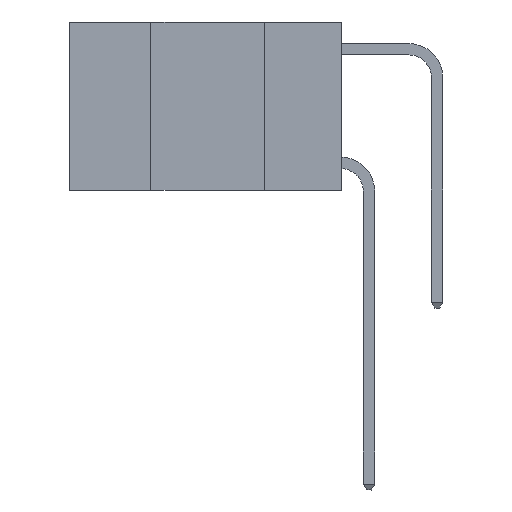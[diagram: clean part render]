
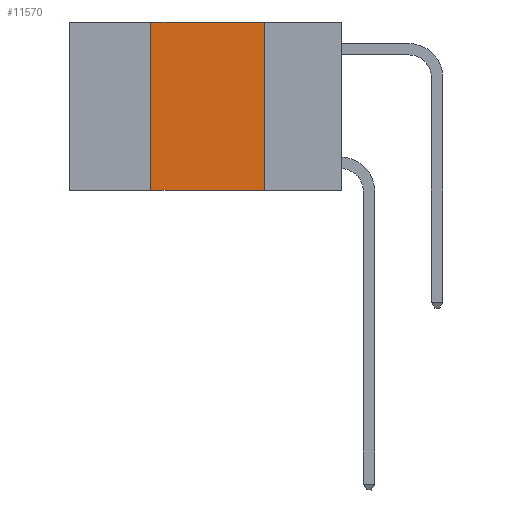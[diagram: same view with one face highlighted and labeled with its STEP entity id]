
A CAD part, left-side view. The second image highlights one B-rep face of the part: STEP entity #11570.
In plain terms, the highlighted planar face has unit normal (-1, 0, 0).
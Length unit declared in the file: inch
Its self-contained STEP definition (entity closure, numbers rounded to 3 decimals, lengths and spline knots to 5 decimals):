
#505 = VERTEX_POINT ( 'NONE', #12590 ) ;
#837 = VERTEX_POINT ( 'NONE', #8131 ) ;
#1138 = CARTESIAN_POINT ( 'NONE',  ( 0., 0.6, 0. ) ) ;
#1739 = LINE ( 'NONE', #2656, #2370 ) ;
#2370 = VECTOR ( 'NONE', #2775, 39.37008 ) ;
#2593 = ORIENTED_EDGE ( 'NONE', *, *, #11526, .T. ) ;
#2656 = CARTESIAN_POINT ( 'NONE',  ( 0., 0.6, -0.37 ) ) ;
#2663 = ORIENTED_EDGE ( 'NONE', *, *, #3154, .F. ) ;
#2713 = CARTESIAN_POINT ( 'NONE',  ( 0., 0.6, 0. ) ) ;
#2775 = DIRECTION ( 'NONE',  ( 0., -1., 0. ) ) ;
#2803 = VERTEX_POINT ( 'NONE', #5694 ) ;
#2835 = CARTESIAN_POINT ( 'NONE',  ( 0., 0.17, 0. ) ) ;
#3154 = EDGE_CURVE ( 'NONE', #2803, #837, #12061, .T. ) ;
#3201 = EDGE_LOOP ( 'NONE', ( #5279, #2663, #4880, #2593 ) ) ;
#3509 = VECTOR ( 'NONE', #8747, 39.37008 ) ;
#3903 = CARTESIAN_POINT ( 'NONE',  ( 0., 0.42, 0. ) ) ;
#4802 = DIRECTION ( 'NONE',  ( 1., 0., 0. ) ) ;
#4880 = ORIENTED_EDGE ( 'NONE', *, *, #4942, .F. ) ;
#4942 = EDGE_CURVE ( 'NONE', #10172, #2803, #7715, .T. ) ;
#4985 = VECTOR ( 'NONE', #5083, 39.37008 ) ;
#5083 = DIRECTION ( 'NONE',  ( 0., -1., 0. ) ) ;
#5279 = ORIENTED_EDGE ( 'NONE', *, *, #10167, .F. ) ;
#5694 = CARTESIAN_POINT ( 'NONE',  ( 0., 0.42, 0. ) ) ;
#6805 = FACE_OUTER_BOUND ( 'NONE', #3201, .T. ) ;
#7715 = LINE ( 'NONE', #3903, #3509 ) ;
#7814 = LINE ( 'NONE', #2835, #8498 ) ;
#8131 = CARTESIAN_POINT ( 'NONE',  ( 0., 0.17, 0. ) ) ;
#8498 = VECTOR ( 'NONE', #9547, 39.37008 ) ;
#8747 = DIRECTION ( 'NONE',  ( 0., 0., 1. ) ) ;
#9547 = DIRECTION ( 'NONE',  ( 0., 0., -1. ) ) ;
#10167 = EDGE_CURVE ( 'NONE', #837, #505, #7814, .T. ) ;
#10172 = VERTEX_POINT ( 'NONE', #10623 ) ;
#10623 = CARTESIAN_POINT ( 'NONE',  ( 0., 0.42, -0.37 ) ) ;
#10689 = PLANE ( 'NONE',  #12362 ) ;
#11526 = EDGE_CURVE ( 'NONE', #10172, #505, #1739, .T. ) ;
#11570 = ADVANCED_FACE ( 'NONE', ( #6805 ), #10689, .F. ) ;
#12061 = LINE ( 'NONE', #1138, #4985 ) ;
#12362 = AXIS2_PLACEMENT_3D ( 'NONE', #2713, #4802, #12411 ) ;
#12411 = DIRECTION ( 'NONE',  ( 0., 0., -1. ) ) ;
#12590 = CARTESIAN_POINT ( 'NONE',  ( 0., 0.17, -0.37 ) ) ;
